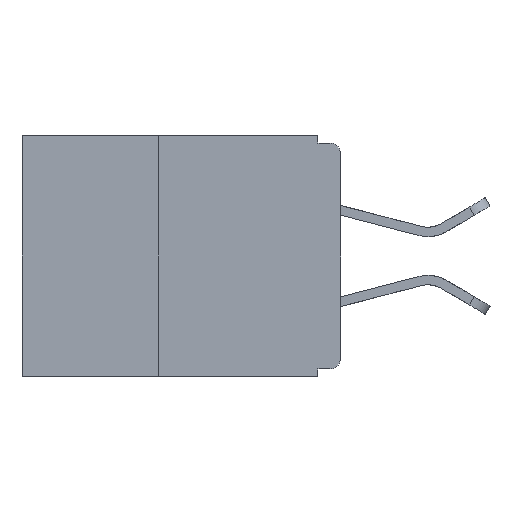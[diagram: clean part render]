
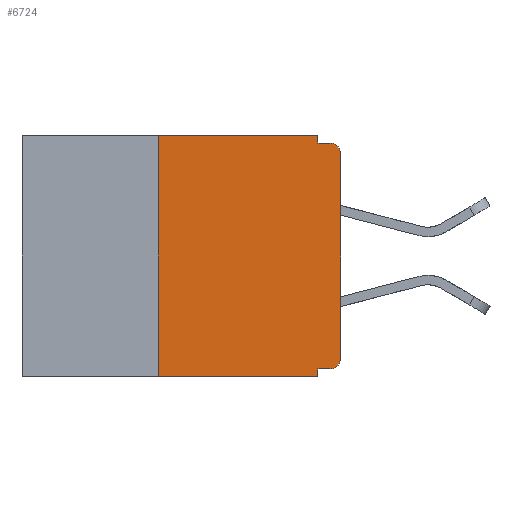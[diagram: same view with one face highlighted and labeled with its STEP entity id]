
A CAD part, left-side view. The second image highlights one B-rep face of the part: STEP entity #6724.
In plain terms, the highlighted planar face has unit normal (-1, 0, 0).
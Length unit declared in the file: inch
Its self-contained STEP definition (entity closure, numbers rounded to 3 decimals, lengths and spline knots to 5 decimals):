
#359 = VERTEX_POINT ( 'NONE', #9640 ) ;
#737 = CARTESIAN_POINT ( 'NONE',  ( 0., 0.437, 0. ) ) ;
#798 = VERTEX_POINT ( 'NONE', #13151 ) ;
#1051 = EDGE_CURVE ( 'NONE', #13894, #11786, #17578, .T. ) ;
#1495 = VERTEX_POINT ( 'NONE', #7150 ) ;
#1570 = ORIENTED_EDGE ( 'NONE', *, *, #3233, .F. ) ;
#1644 = AXIS2_PLACEMENT_3D ( 'NONE', #8195, #8510, #8443 ) ;
#1885 = EDGE_CURVE ( 'NONE', #11786, #11229, #4724, .T. ) ;
#2089 = CARTESIAN_POINT ( 'NONE',  ( 0., 0.031, -0.01 ) ) ;
#2276 = EDGE_CURVE ( 'NONE', #9036, #15415, #10601, .T. ) ;
#2615 = CARTESIAN_POINT ( 'NONE',  ( 0., 0.015, -0.01 ) ) ;
#3118 = ORIENTED_EDGE ( 'NONE', *, *, #10554, .T. ) ;
#3233 = EDGE_CURVE ( 'NONE', #8400, #359, #5400, .T. ) ;
#4199 = LINE ( 'NONE', #11218, #19311 ) ;
#4724 = CIRCLE ( 'NONE', #14802, 0.015 ) ;
#4726 = DIRECTION ( 'NONE',  ( 0., -1., 0. ) ) ;
#4981 = VECTOR ( 'NONE', #17497, 39.37008 ) ;
#5022 = FACE_OUTER_BOUND ( 'NONE', #11412, .T. ) ;
#5200 = ORIENTED_EDGE ( 'NONE', *, *, #1885, .T. ) ;
#5400 = LINE ( 'NONE', #737, #8915 ) ;
#5971 = DIRECTION ( 'NONE',  ( -1., 0., 0. ) ) ;
#6194 = VECTOR ( 'NONE', #11007, 39.37008 ) ;
#6423 = DIRECTION ( 'NONE',  ( 0., 0., -1. ) ) ;
#6444 = DIRECTION ( 'NONE',  ( -1., 0., 0. ) ) ;
#6506 = CARTESIAN_POINT ( 'NONE',  ( 0., 0.015, -0.305 ) ) ;
#6651 = DIRECTION ( 'NONE',  ( 0., 0., 1. ) ) ;
#6724 = ADVANCED_FACE ( 'NONE', ( #5022 ), #7957, .F. ) ;
#6848 = ORIENTED_EDGE ( 'NONE', *, *, #7215, .F. ) ;
#7150 = CARTESIAN_POINT ( 'NONE',  ( 0., 0.031, -0.32 ) ) ;
#7215 = EDGE_CURVE ( 'NONE', #798, #1495, #11583, .T. ) ;
#7557 = EDGE_CURVE ( 'NONE', #9036, #8400, #16677, .T. ) ;
#7667 = CARTESIAN_POINT ( 'NONE',  ( 0., 0.031, 0. ) ) ;
#7744 = DIRECTION ( 'NONE',  ( 0., 0., -1. ) ) ;
#7846 = EDGE_CURVE ( 'NONE', #13553, #11229, #4199, .T. ) ;
#7957 = PLANE ( 'NONE',  #1644 ) ;
#8195 = CARTESIAN_POINT ( 'NONE',  ( 0., 0.437, 0. ) ) ;
#8280 = ORIENTED_EDGE ( 'NONE', *, *, #7846, .F. ) ;
#8400 = VERTEX_POINT ( 'NONE', #17996 ) ;
#8443 = DIRECTION ( 'NONE',  ( 0., 0., -1. ) ) ;
#8510 = DIRECTION ( 'NONE',  ( 1., 0., 0. ) ) ;
#8915 = VECTOR ( 'NONE', #4726, 39.37008 ) ;
#9036 = VERTEX_POINT ( 'NONE', #12334 ) ;
#9125 = DIRECTION ( 'NONE',  ( 0., 0., -1. ) ) ;
#9242 = CARTESIAN_POINT ( 'NONE',  ( 0., 0.031, -0.33 ) ) ;
#9539 = EDGE_CURVE ( 'NONE', #359, #13553, #9572, .T. ) ;
#9572 = LINE ( 'NONE', #7667, #16783 ) ;
#9640 = CARTESIAN_POINT ( 'NONE',  ( 0., 0.031, 0. ) ) ;
#10295 = ORIENTED_EDGE ( 'NONE', *, *, #9539, .F. ) ;
#10554 = EDGE_CURVE ( 'NONE', #798, #13894, #14985, .T. ) ;
#10601 = LINE ( 'NONE', #11565, #6194 ) ;
#11007 = DIRECTION ( 'NONE',  ( 0., -1., 0. ) ) ;
#11218 = CARTESIAN_POINT ( 'NONE',  ( 0., 0., -0.01 ) ) ;
#11229 = VERTEX_POINT ( 'NONE', #2615 ) ;
#11329 = DIRECTION ( 'NONE',  ( 0., -1., 0. ) ) ;
#11412 = EDGE_LOOP ( 'NONE', ( #19022, #5200, #8280, #10295, #1570, #17921, #15927, #12646, #6848, #3118 ) ) ;
#11445 = CARTESIAN_POINT ( 'NONE',  ( 0., 0.031, -0.33 ) ) ;
#11565 = CARTESIAN_POINT ( 'NONE',  ( 0., 0.437, -0.33 ) ) ;
#11574 = CARTESIAN_POINT ( 'NONE',  ( 0., 0., 0. ) ) ;
#11583 = LINE ( 'NONE', #11841, #15357 ) ;
#11755 = DIRECTION ( 'NONE',  ( 0., 1., 0. ) ) ;
#11786 = VERTEX_POINT ( 'NONE', #12696 ) ;
#11841 = CARTESIAN_POINT ( 'NONE',  ( 0., 0., -0.32 ) ) ;
#12334 = CARTESIAN_POINT ( 'NONE',  ( 0., 0.25, -0.33 ) ) ;
#12519 = AXIS2_PLACEMENT_3D ( 'NONE', #6506, #6444, #6423 ) ;
#12646 = ORIENTED_EDGE ( 'NONE', *, *, #18539, .F. ) ;
#12696 = CARTESIAN_POINT ( 'NONE',  ( 0., 0., -0.025 ) ) ;
#13151 = CARTESIAN_POINT ( 'NONE',  ( 0., 0.015, -0.32 ) ) ;
#13321 = CARTESIAN_POINT ( 'NONE',  ( 0., 0.015, -0.025 ) ) ;
#13553 = VERTEX_POINT ( 'NONE', #2089 ) ;
#13894 = VERTEX_POINT ( 'NONE', #16272 ) ;
#14686 = VECTOR ( 'NONE', #19290, 39.37008 ) ;
#14734 = VECTOR ( 'NONE', #6651, 39.37008 ) ;
#14802 = AXIS2_PLACEMENT_3D ( 'NONE', #13321, #5971, #9125 ) ;
#14985 = CIRCLE ( 'NONE', #12519, 0.015 ) ;
#15357 = VECTOR ( 'NONE', #11755, 39.37008 ) ;
#15415 = VERTEX_POINT ( 'NONE', #11445 ) ;
#15927 = ORIENTED_EDGE ( 'NONE', *, *, #2276, .T. ) ;
#16272 = CARTESIAN_POINT ( 'NONE',  ( 0., 0., -0.305 ) ) ;
#16677 = LINE ( 'NONE', #17709, #4981 ) ;
#16783 = VECTOR ( 'NONE', #7744, 39.37008 ) ;
#17497 = DIRECTION ( 'NONE',  ( 0., 0., 1. ) ) ;
#17578 = LINE ( 'NONE', #11574, #14734 ) ;
#17709 = CARTESIAN_POINT ( 'NONE',  ( 0., 0.25, -0.33 ) ) ;
#17921 = ORIENTED_EDGE ( 'NONE', *, *, #7557, .F. ) ;
#17972 = LINE ( 'NONE', #9242, #14686 ) ;
#17996 = CARTESIAN_POINT ( 'NONE',  ( 0., 0.25, 0. ) ) ;
#18539 = EDGE_CURVE ( 'NONE', #1495, #15415, #17972, .T. ) ;
#19022 = ORIENTED_EDGE ( 'NONE', *, *, #1051, .T. ) ;
#19290 = DIRECTION ( 'NONE',  ( 0., 0., -1. ) ) ;
#19311 = VECTOR ( 'NONE', #11329, 39.37008 ) ;
